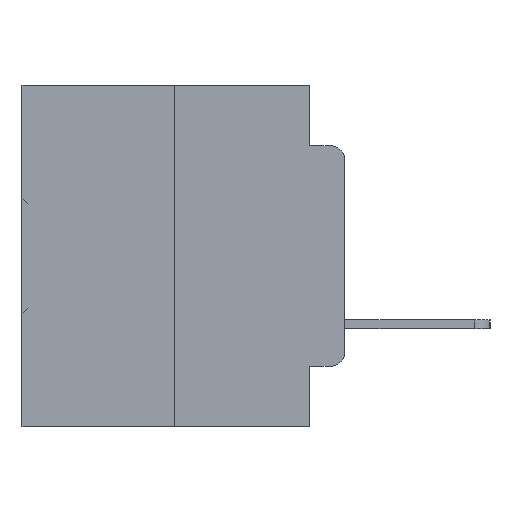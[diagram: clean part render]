
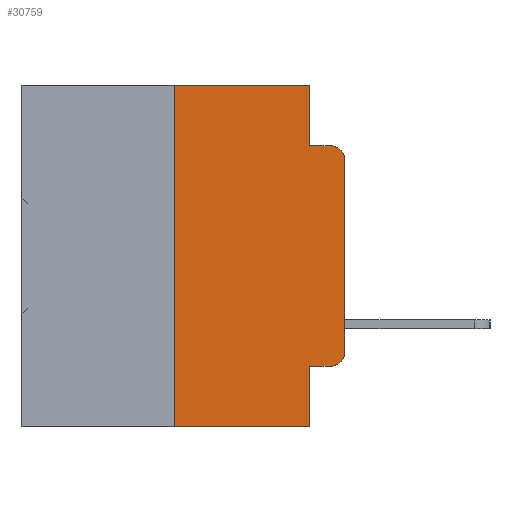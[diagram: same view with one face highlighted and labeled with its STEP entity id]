
A CAD part, left-side view. The second image highlights one B-rep face of the part: STEP entity #30759.
In plain terms, the highlighted planar face has unit normal (-1, 0, 0).
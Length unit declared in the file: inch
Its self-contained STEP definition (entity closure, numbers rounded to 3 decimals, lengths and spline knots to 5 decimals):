
#359 = CARTESIAN_POINT ( 'NONE',  ( 0., 0.02, -0.3915 ) ) ;
#377 = DIRECTION ( 'NONE',  ( 0., -1., 0. ) ) ;
#1231 = EDGE_CURVE ( 'NONE', #6488, #27605, #8568, .T. ) ;
#1257 = LINE ( 'NONE', #21278, #21689 ) ;
#1323 = VECTOR ( 'NONE', #377, 39.37008 ) ;
#1428 = EDGE_LOOP ( 'NONE', ( #4811, #13685, #23263, #1793, #33249, #6877, #9046, #26946, #27004, #9453 ) ) ;
#1793 = ORIENTED_EDGE ( 'NONE', *, *, #17183, .F. ) ;
#1836 = DIRECTION ( 'NONE',  ( 0., -1., 0. ) ) ;
#2112 = LINE ( 'NONE', #18324, #15575 ) ;
#2879 = EDGE_CURVE ( 'NONE', #13093, #6488, #10619, .T. ) ;
#3148 = DIRECTION ( 'NONE',  ( 0., 0., -1. ) ) ;
#3502 = VERTEX_POINT ( 'NONE', #9309 ) ;
#3737 = DIRECTION ( 'NONE',  ( 0., -1., 0. ) ) ;
#4558 = VECTOR ( 'NONE', #22477, 39.37008 ) ;
#4811 = ORIENTED_EDGE ( 'NONE', *, *, #18548, .T. ) ;
#4963 = CARTESIAN_POINT ( 'NONE',  ( 0., 0.02, -0.4115 ) ) ;
#5048 = LINE ( 'NONE', #33123, #17462 ) ;
#5856 = AXIS2_PLACEMENT_3D ( 'NONE', #359, #19093, #3148 ) ;
#6488 = VERTEX_POINT ( 'NONE', #18123 ) ;
#6577 = CARTESIAN_POINT ( 'NONE',  ( 0., 0.02, -0.1085 ) ) ;
#6642 = DIRECTION ( 'NONE',  ( 1., 0., 0. ) ) ;
#6703 = CARTESIAN_POINT ( 'NONE',  ( 0., 0.02, -0.0885 ) ) ;
#6877 = ORIENTED_EDGE ( 'NONE', *, *, #2879, .F. ) ;
#7810 = DIRECTION ( 'NONE',  ( 0., 0., -1. ) ) ;
#8407 = CARTESIAN_POINT ( 'NONE',  ( 0., 0., 0. ) ) ;
#8568 = LINE ( 'NONE', #13678, #1323 ) ;
#9046 = ORIENTED_EDGE ( 'NONE', *, *, #21103, .T. ) ;
#9309 = CARTESIAN_POINT ( 'NONE',  ( 0., 0.051, -0.5 ) ) ;
#9324 = DIRECTION ( 'NONE',  ( 0., 0., -1. ) ) ;
#9331 = CARTESIAN_POINT ( 'NONE',  ( 0., 0.051, -0.0885 ) ) ;
#9453 = ORIENTED_EDGE ( 'NONE', *, *, #16134, .T. ) ;
#10619 = LINE ( 'NONE', #28808, #24418 ) ;
#12013 = CARTESIAN_POINT ( 'NONE',  ( 0., 0.473, 0. ) ) ;
#12235 = CARTESIAN_POINT ( 'NONE',  ( 0., 0.25, -0.5 ) ) ;
#12589 = LINE ( 'NONE', #9331, #4558 ) ;
#13093 = VERTEX_POINT ( 'NONE', #12235 ) ;
#13678 = CARTESIAN_POINT ( 'NONE',  ( 0., 0.473, 0. ) ) ;
#13685 = ORIENTED_EDGE ( 'NONE', *, *, #30124, .T. ) ;
#13711 = VERTEX_POINT ( 'NONE', #6703 ) ;
#14446 = CIRCLE ( 'NONE', #5856, 0.02 ) ;
#15397 = AXIS2_PLACEMENT_3D ( 'NONE', #12013, #6642, #25005 ) ;
#15575 = VECTOR ( 'NONE', #7810, 39.37008 ) ;
#16134 = EDGE_CURVE ( 'NONE', #32642, #30366, #14446, .T. ) ;
#16427 = VERTEX_POINT ( 'NONE', #32966 ) ;
#17183 = EDGE_CURVE ( 'NONE', #27605, #23377, #2112, .T. ) ;
#17462 = VECTOR ( 'NONE', #1836, 39.37008 ) ;
#18123 = CARTESIAN_POINT ( 'NONE',  ( 0., 0.25, 0. ) ) ;
#18324 = CARTESIAN_POINT ( 'NONE',  ( 0., 0.051, 0. ) ) ;
#18548 = EDGE_CURVE ( 'NONE', #30366, #16427, #29336, .T. ) ;
#19030 = DIRECTION ( 'NONE',  ( 0., 0., 1. ) ) ;
#19093 = DIRECTION ( 'NONE',  ( -1., 0., 0. ) ) ;
#19655 = CARTESIAN_POINT ( 'NONE',  ( 0., 0.473, -0.5 ) ) ;
#21103 = EDGE_CURVE ( 'NONE', #13093, #3502, #31531, .T. ) ;
#21278 = CARTESIAN_POINT ( 'NONE',  ( 0., 0.051, 0. ) ) ;
#21337 = EDGE_CURVE ( 'NONE', #25384, #32642, #5048, .T. ) ;
#21689 = VECTOR ( 'NONE', #23843, 39.37008 ) ;
#21719 = CARTESIAN_POINT ( 'NONE',  ( 0., 0.051, -0.0885 ) ) ;
#22477 = DIRECTION ( 'NONE',  ( 0., -1., 0. ) ) ;
#22544 = VECTOR ( 'NONE', #19030, 39.37008 ) ;
#22960 = CARTESIAN_POINT ( 'NONE',  ( 0., 0.051, 0. ) ) ;
#23263 = ORIENTED_EDGE ( 'NONE', *, *, #31829, .F. ) ;
#23377 = VERTEX_POINT ( 'NONE', #21719 ) ;
#23843 = DIRECTION ( 'NONE',  ( 0., 0., -1. ) ) ;
#24418 = VECTOR ( 'NONE', #28838, 39.37008 ) ;
#24928 = DIRECTION ( 'NONE',  ( -1., 0., 0. ) ) ;
#25005 = DIRECTION ( 'NONE',  ( 0., 0., -1. ) ) ;
#25384 = VERTEX_POINT ( 'NONE', #29915 ) ;
#25577 = VECTOR ( 'NONE', #3737, 39.37008 ) ;
#26946 = ORIENTED_EDGE ( 'NONE', *, *, #29865, .F. ) ;
#27004 = ORIENTED_EDGE ( 'NONE', *, *, #21337, .T. ) ;
#27605 = VERTEX_POINT ( 'NONE', #22960 ) ;
#27653 = AXIS2_PLACEMENT_3D ( 'NONE', #6577, #24928, #9324 ) ;
#28402 = FACE_OUTER_BOUND ( 'NONE', #1428, .T. ) ;
#28808 = CARTESIAN_POINT ( 'NONE',  ( 0., 0.25, 0. ) ) ;
#28838 = DIRECTION ( 'NONE',  ( 0., 0., 1. ) ) ;
#29336 = LINE ( 'NONE', #8407, #22544 ) ;
#29865 = EDGE_CURVE ( 'NONE', #25384, #3502, #1257, .T. ) ;
#29915 = CARTESIAN_POINT ( 'NONE',  ( 0., 0.051, -0.4115 ) ) ;
#30124 = EDGE_CURVE ( 'NONE', #16427, #13711, #33960, .T. ) ;
#30366 = VERTEX_POINT ( 'NONE', #31040 ) ;
#30759 = ADVANCED_FACE ( 'NONE', ( #28402 ), #32523, .F. ) ;
#31040 = CARTESIAN_POINT ( 'NONE',  ( 0., 0., -0.3915 ) ) ;
#31531 = LINE ( 'NONE', #19655, #25577 ) ;
#31829 = EDGE_CURVE ( 'NONE', #23377, #13711, #12589, .T. ) ;
#32523 = PLANE ( 'NONE',  #15397 ) ;
#32642 = VERTEX_POINT ( 'NONE', #4963 ) ;
#32966 = CARTESIAN_POINT ( 'NONE',  ( 0., 0., -0.1085 ) ) ;
#33123 = CARTESIAN_POINT ( 'NONE',  ( 0., 0.051, -0.4115 ) ) ;
#33249 = ORIENTED_EDGE ( 'NONE', *, *, #1231, .F. ) ;
#33960 = CIRCLE ( 'NONE', #27653, 0.02 ) ;
